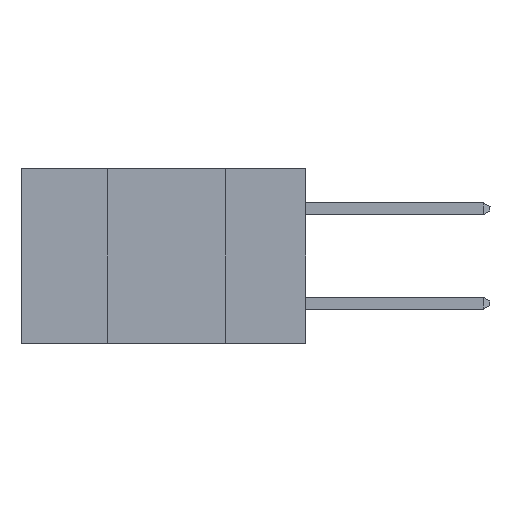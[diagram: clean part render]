
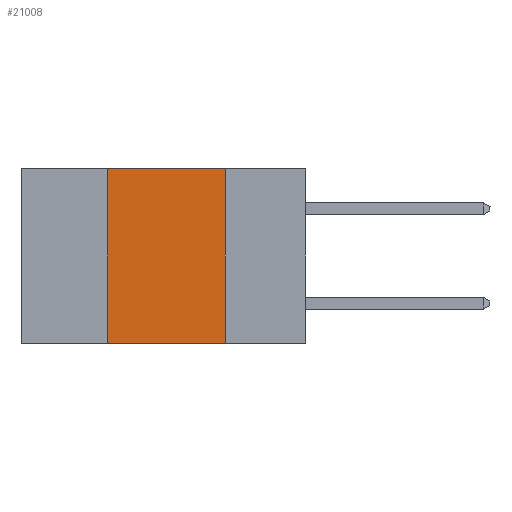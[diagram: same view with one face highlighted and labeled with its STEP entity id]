
A CAD part, left-side view. The second image highlights one B-rep face of the part: STEP entity #21008.
In plain terms, the highlighted planar face has unit normal (-1, 0, 0).
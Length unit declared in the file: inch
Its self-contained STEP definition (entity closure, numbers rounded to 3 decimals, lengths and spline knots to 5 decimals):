
#494 = VECTOR ( 'NONE', #14004, 39.37008 ) ;
#987 = VECTOR ( 'NONE', #22100, 39.37008 ) ;
#2194 = PLANE ( 'NONE',  #14126 ) ;
#2278 = FACE_OUTER_BOUND ( 'NONE', #32641, .T. ) ;
#2602 = VECTOR ( 'NONE', #9466, 39.37008 ) ;
#2641 = CARTESIAN_POINT ( 'NONE',  ( 0., 0.6, 0. ) ) ;
#3449 = LINE ( 'NONE', #19842, #2602 ) ;
#3488 = EDGE_CURVE ( 'NONE', #28452, #12101, #3449, .T. ) ;
#5747 = VERTEX_POINT ( 'NONE', #23325 ) ;
#8724 = ORIENTED_EDGE ( 'NONE', *, *, #3488, .F. ) ;
#9466 = DIRECTION ( 'NONE',  ( 0., 0., 1. ) ) ;
#10098 = DIRECTION ( 'NONE',  ( 1., 0., 0. ) ) ;
#11467 = CARTESIAN_POINT ( 'NONE',  ( 0., 0.17, 0. ) ) ;
#12101 = VERTEX_POINT ( 'NONE', #30440 ) ;
#12857 = EDGE_CURVE ( 'NONE', #12101, #5747, #25481, .T. ) ;
#13804 = ORIENTED_EDGE ( 'NONE', *, *, #19658, .T. ) ;
#14004 = DIRECTION ( 'NONE',  ( 0., -1., 0. ) ) ;
#14126 = AXIS2_PLACEMENT_3D ( 'NONE', #2641, #10098, #28944 ) ;
#15876 = CARTESIAN_POINT ( 'NONE',  ( 0., 0.17, -0.37 ) ) ;
#17112 = CARTESIAN_POINT ( 'NONE',  ( 0., 0.42, -0.37 ) ) ;
#18358 = EDGE_CURVE ( 'NONE', #5747, #18692, #24752, .T. ) ;
#18692 = VERTEX_POINT ( 'NONE', #15876 ) ;
#19431 = VECTOR ( 'NONE', #20826, 39.37008 ) ;
#19658 = EDGE_CURVE ( 'NONE', #28452, #18692, #26117, .T. ) ;
#19842 = CARTESIAN_POINT ( 'NONE',  ( 0., 0.42, 0. ) ) ;
#20826 = DIRECTION ( 'NONE',  ( 0., -1., 0. ) ) ;
#21008 = ADVANCED_FACE ( 'NONE', ( #2278 ), #2194, .F. ) ;
#22100 = DIRECTION ( 'NONE',  ( 0., 0., -1. ) ) ;
#23325 = CARTESIAN_POINT ( 'NONE',  ( 0., 0.17, 0. ) ) ;
#24288 = CARTESIAN_POINT ( 'NONE',  ( 0., 0.6, 0. ) ) ;
#24752 = LINE ( 'NONE', #11467, #987 ) ;
#25481 = LINE ( 'NONE', #24288, #494 ) ;
#26117 = LINE ( 'NONE', #34046, #19431 ) ;
#28452 = VERTEX_POINT ( 'NONE', #17112 ) ;
#28944 = DIRECTION ( 'NONE',  ( 0., 0., -1. ) ) ;
#29476 = ORIENTED_EDGE ( 'NONE', *, *, #18358, .F. ) ;
#30407 = ORIENTED_EDGE ( 'NONE', *, *, #12857, .F. ) ;
#30440 = CARTESIAN_POINT ( 'NONE',  ( 0., 0.42, 0. ) ) ;
#32641 = EDGE_LOOP ( 'NONE', ( #29476, #30407, #8724, #13804 ) ) ;
#34046 = CARTESIAN_POINT ( 'NONE',  ( 0., 0.6, -0.37 ) ) ;
